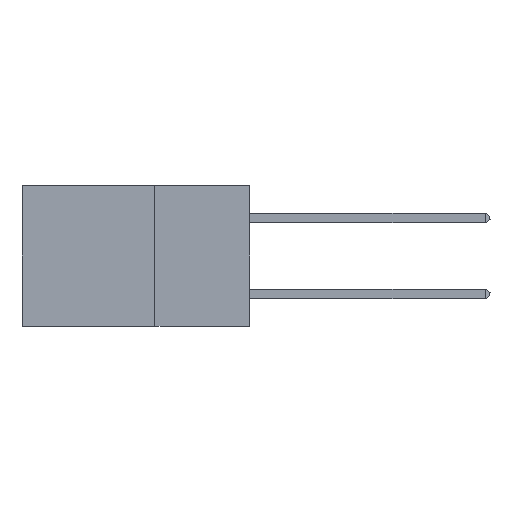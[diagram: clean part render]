
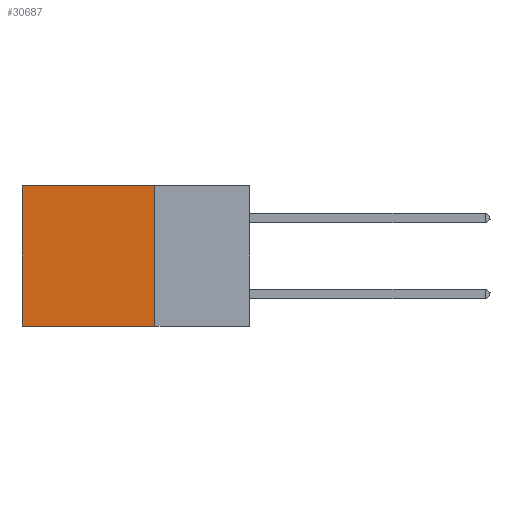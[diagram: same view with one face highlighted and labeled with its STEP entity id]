
A CAD part, left-side view. The second image highlights one B-rep face of the part: STEP entity #30687.
In plain terms, the highlighted planar face has unit normal (-1, 0, 0).
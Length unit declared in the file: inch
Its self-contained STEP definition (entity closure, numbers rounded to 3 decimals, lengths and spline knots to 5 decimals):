
#80 = ORIENTED_EDGE ( 'NONE', *, *, #16092, .F. ) ;
#4415 = CARTESIAN_POINT ( 'NONE',  ( 0.2875, 0.25, 0. ) ) ;
#4588 = EDGE_LOOP ( 'NONE', ( #19151, #23903, #80, #22998 ) ) ;
#5299 = LINE ( 'NONE', #29657, #18056 ) ;
#5455 = EDGE_CURVE ( 'NONE', #18193, #5498, #5299, .T. ) ;
#5498 = VERTEX_POINT ( 'NONE', #15501 ) ;
#6473 = VECTOR ( 'NONE', #27399, 39.37008 ) ;
#7225 = LINE ( 'NONE', #25048, #6473 ) ;
#9303 = EDGE_CURVE ( 'NONE', #18656, #28860, #7225, .T. ) ;
#9965 = CARTESIAN_POINT ( 'NONE',  ( 0.2875, 0.6, 0. ) ) ;
#12313 = DIRECTION ( 'NONE',  ( 0., 0., -1. ) ) ;
#12843 = VECTOR ( 'NONE', #12313, 39.37008 ) ;
#13088 = DIRECTION ( 'NONE',  ( 0., 1., 0. ) ) ;
#13165 = AXIS2_PLACEMENT_3D ( 'NONE', #4415, #30596, #16453 ) ;
#14411 = CARTESIAN_POINT ( 'NONE',  ( 0.2875, 0.25, 0. ) ) ;
#15501 = CARTESIAN_POINT ( 'NONE',  ( 0.2875, 0.6, -0.37 ) ) ;
#15709 = CARTESIAN_POINT ( 'NONE',  ( 0.2875, 0.25, 0. ) ) ;
#16092 = EDGE_CURVE ( 'NONE', #18656, #18193, #21547, .T. ) ;
#16453 = DIRECTION ( 'NONE',  ( 0., 0., -1. ) ) ;
#16820 = DIRECTION ( 'NONE',  ( 0., 0., -1. ) ) ;
#18056 = VECTOR ( 'NONE', #13088, 39.37008 ) ;
#18193 = VERTEX_POINT ( 'NONE', #28249 ) ;
#18256 = FACE_OUTER_BOUND ( 'NONE', #4588, .T. ) ;
#18656 = VERTEX_POINT ( 'NONE', #15709 ) ;
#19151 = ORIENTED_EDGE ( 'NONE', *, *, #24512, .T. ) ;
#19203 = LINE ( 'NONE', #9965, #12843 ) ;
#20803 = VECTOR ( 'NONE', #16820, 39.37008 ) ;
#21547 = LINE ( 'NONE', #14411, #20803 ) ;
#22998 = ORIENTED_EDGE ( 'NONE', *, *, #9303, .T. ) ;
#23903 = ORIENTED_EDGE ( 'NONE', *, *, #5455, .F. ) ;
#24512 = EDGE_CURVE ( 'NONE', #28860, #5498, #19203, .T. ) ;
#25048 = CARTESIAN_POINT ( 'NONE',  ( 0.2875, 0.25, 0. ) ) ;
#27399 = DIRECTION ( 'NONE',  ( 0., 1., 0. ) ) ;
#27463 = CARTESIAN_POINT ( 'NONE',  ( 0.2875, 0.6, 0. ) ) ;
#28232 = PLANE ( 'NONE',  #13165 ) ;
#28249 = CARTESIAN_POINT ( 'NONE',  ( 0.2875, 0.25, -0.37 ) ) ;
#28860 = VERTEX_POINT ( 'NONE', #27463 ) ;
#29657 = CARTESIAN_POINT ( 'NONE',  ( 0.2875, 0.25, -0.37 ) ) ;
#30596 = DIRECTION ( 'NONE',  ( 1., 0., 0. ) ) ;
#30687 = ADVANCED_FACE ( 'NONE', ( #18256 ), #28232, .F. ) ;
